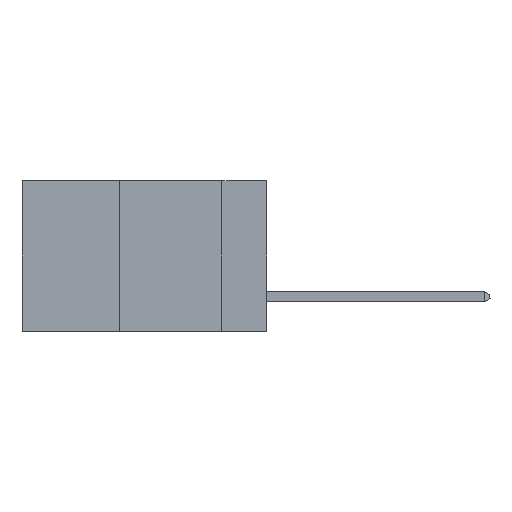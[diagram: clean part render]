
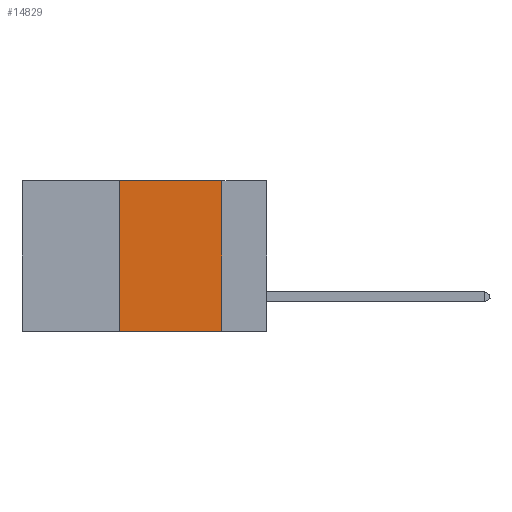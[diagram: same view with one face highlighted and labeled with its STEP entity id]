
A CAD part, left-side view. The second image highlights one B-rep face of the part: STEP entity #14829.
In plain terms, the highlighted planar face has unit normal (-1, 0, 0).
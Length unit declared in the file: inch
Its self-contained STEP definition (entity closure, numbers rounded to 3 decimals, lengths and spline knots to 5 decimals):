
#468 = LINE ( 'NONE', #2879, #37934 ) ;
#2169 = CARTESIAN_POINT ( 'NONE',  ( 0., 0.11, -0.37 ) ) ;
#2879 = CARTESIAN_POINT ( 'NONE',  ( 0., 0.36, 0. ) ) ;
#5122 = DIRECTION ( 'NONE',  ( 1., 0., 0. ) ) ;
#6004 = CARTESIAN_POINT ( 'NONE',  ( 0., 0.11, 0. ) ) ;
#7444 = VECTOR ( 'NONE', #8446, 39.37008 ) ;
#8440 = CARTESIAN_POINT ( 'NONE',  ( 0., 0.6, 0. ) ) ;
#8446 = DIRECTION ( 'NONE',  ( 0., -1., 0. ) ) ;
#9055 = DIRECTION ( 'NONE',  ( 0., -1., 0. ) ) ;
#9854 = EDGE_CURVE ( 'NONE', #9879, #11818, #468, .T. ) ;
#9879 = VERTEX_POINT ( 'NONE', #27418 ) ;
#9898 = EDGE_CURVE ( 'NONE', #9879, #20466, #11087, .T. ) ;
#10215 = VERTEX_POINT ( 'NONE', #6004 ) ;
#10798 = ORIENTED_EDGE ( 'NONE', *, *, #20025, .F. ) ;
#11087 = LINE ( 'NONE', #33040, #38402 ) ;
#11307 = DIRECTION ( 'NONE',  ( 0., 0., -1. ) ) ;
#11818 = VERTEX_POINT ( 'NONE', #22031 ) ;
#12628 = EDGE_CURVE ( 'NONE', #11818, #10215, #17564, .T. ) ;
#12897 = VECTOR ( 'NONE', #33113, 39.37008 ) ;
#14829 = ADVANCED_FACE ( 'NONE', ( #27465 ), #17341, .F. ) ;
#17341 = PLANE ( 'NONE',  #25139 ) ;
#17564 = LINE ( 'NONE', #35916, #7444 ) ;
#19552 = EDGE_LOOP ( 'NONE', ( #10798, #33099, #25574, #21418 ) ) ;
#20025 = EDGE_CURVE ( 'NONE', #10215, #20466, #27254, .T. ) ;
#20466 = VERTEX_POINT ( 'NONE', #2169 ) ;
#21418 = ORIENTED_EDGE ( 'NONE', *, *, #9898, .T. ) ;
#22031 = CARTESIAN_POINT ( 'NONE',  ( 0., 0.36, 0. ) ) ;
#25139 = AXIS2_PLACEMENT_3D ( 'NONE', #8440, #5122, #11307 ) ;
#25574 = ORIENTED_EDGE ( 'NONE', *, *, #9854, .F. ) ;
#27254 = LINE ( 'NONE', #30164, #12897 ) ;
#27418 = CARTESIAN_POINT ( 'NONE',  ( 0., 0.36, -0.37 ) ) ;
#27465 = FACE_OUTER_BOUND ( 'NONE', #19552, .T. ) ;
#30164 = CARTESIAN_POINT ( 'NONE',  ( 0., 0.11, 0. ) ) ;
#33040 = CARTESIAN_POINT ( 'NONE',  ( 0., 0.6, -0.37 ) ) ;
#33099 = ORIENTED_EDGE ( 'NONE', *, *, #12628, .F. ) ;
#33113 = DIRECTION ( 'NONE',  ( 0., 0., -1. ) ) ;
#33436 = DIRECTION ( 'NONE',  ( 0., 0., 1. ) ) ;
#35916 = CARTESIAN_POINT ( 'NONE',  ( 0., 0.6, 0. ) ) ;
#37934 = VECTOR ( 'NONE', #33436, 39.37008 ) ;
#38402 = VECTOR ( 'NONE', #9055, 39.37008 ) ;
